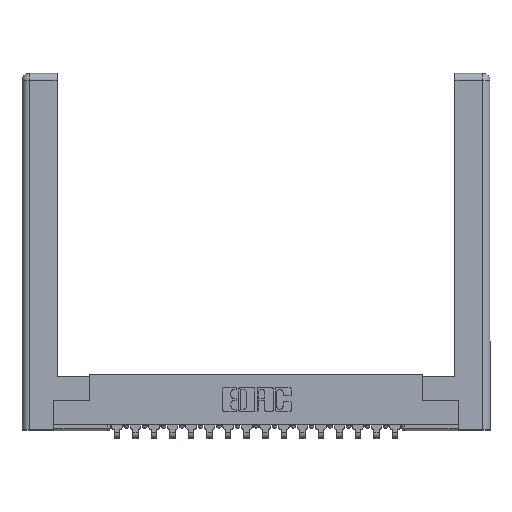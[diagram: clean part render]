
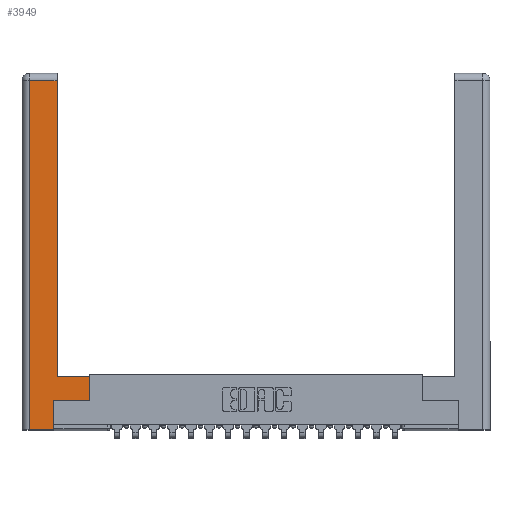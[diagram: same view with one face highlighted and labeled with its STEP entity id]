
A CAD part, top view. The second image highlights one B-rep face of the part: STEP entity #3949.
In plain terms, the highlighted planar face has unit normal (0, 0, 1).
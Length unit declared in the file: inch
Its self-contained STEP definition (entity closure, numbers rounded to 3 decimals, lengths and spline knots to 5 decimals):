
#124 = VECTOR ( 'NONE', #1855, 39.37008 ) ;
#143 = CARTESIAN_POINT ( 'NONE',  ( 0.0615, 2.94, 0. ) ) ;
#228 = VERTEX_POINT ( 'NONE', #16128 ) ;
#897 = EDGE_CURVE ( 'NONE', #4246, #228, #5765, .T. ) ;
#951 = LINE ( 'NONE', #14610, #17757 ) ;
#1146 = EDGE_CURVE ( 'NONE', #18111, #5167, #15781, .T. ) ;
#1274 = CARTESIAN_POINT ( 'NONE',  ( 0.565, 0.45, 0. ) ) ;
#1351 = VECTOR ( 'NONE', #16225, 39.37008 ) ;
#1815 = VERTEX_POINT ( 'NONE', #15613 ) ;
#1855 = DIRECTION ( 'NONE',  ( 0., 1., 0. ) ) ;
#2026 = CARTESIAN_POINT ( 'NONE',  ( 0.265, 0., 0. ) ) ;
#2850 = VECTOR ( 'NONE', #12088, 39.37008 ) ;
#3508 = CARTESIAN_POINT ( 'NONE',  ( 0., 0., 0. ) ) ;
#3619 = EDGE_CURVE ( 'NONE', #10464, #18111, #951, .T. ) ;
#3907 = ORIENTED_EDGE ( 'NONE', *, *, #15767, .T. ) ;
#3949 = ADVANCED_FACE ( 'NONE', ( #6427 ), #17150, .F. ) ;
#4221 = DIRECTION ( 'NONE',  ( 1., 0., 0. ) ) ;
#4240 = VERTEX_POINT ( 'NONE', #12368 ) ;
#4246 = VERTEX_POINT ( 'NONE', #13766 ) ;
#4341 = CARTESIAN_POINT ( 'NONE',  ( 0.265, 0.245, 0. ) ) ;
#4457 = EDGE_LOOP ( 'NONE', ( #18686, #18593, #3907, #13509, #6131, #5398, #11695, #14628 ) ) ;
#4713 = DIRECTION ( 'NONE',  ( -1., 0., 0. ) ) ;
#5167 = VERTEX_POINT ( 'NONE', #4341 ) ;
#5346 = LINE ( 'NONE', #6762, #124 ) ;
#5398 = ORIENTED_EDGE ( 'NONE', *, *, #19373, .T. ) ;
#5441 = DIRECTION ( 'NONE',  ( 0., 1., 0. ) ) ;
#5765 = LINE ( 'NONE', #1274, #13965 ) ;
#5906 = EDGE_CURVE ( 'NONE', #228, #1815, #11993, .T. ) ;
#6131 = ORIENTED_EDGE ( 'NONE', *, *, #1146, .T. ) ;
#6390 = AXIS2_PLACEMENT_3D ( 'NONE', #3508, #12706, #4713 ) ;
#6427 = FACE_OUTER_BOUND ( 'NONE', #4457, .T. ) ;
#6500 = EDGE_CURVE ( 'NONE', #15437, #4240, #12420, .T. ) ;
#6754 = CARTESIAN_POINT ( 'NONE',  ( 0.265, 0.245, 0. ) ) ;
#6762 = CARTESIAN_POINT ( 'NONE',  ( 0.295, 3., 0. ) ) ;
#7241 = DIRECTION ( 'NONE',  ( 1., 0., 0. ) ) ;
#7401 = CARTESIAN_POINT ( 'NONE',  ( 0.295, 0.45, 0. ) ) ;
#9635 = CARTESIAN_POINT ( 'NONE',  ( 0.0615, 0., 0. ) ) ;
#10326 = VECTOR ( 'NONE', #5441, 39.37008 ) ;
#10340 = CARTESIAN_POINT ( 'NONE',  ( 0.565, 0.245, 0. ) ) ;
#10464 = VERTEX_POINT ( 'NONE', #9635 ) ;
#11695 = ORIENTED_EDGE ( 'NONE', *, *, #897, .T. ) ;
#11863 = DIRECTION ( 'NONE',  ( 0., 1., 0. ) ) ;
#11993 = LINE ( 'NONE', #7401, #2850 ) ;
#12088 = DIRECTION ( 'NONE',  ( -1., 0., 0. ) ) ;
#12323 = DIRECTION ( 'NONE',  ( -1., 0., 0. ) ) ;
#12368 = CARTESIAN_POINT ( 'NONE',  ( 0.0615, 2.94, 0. ) ) ;
#12420 = LINE ( 'NONE', #143, #14371 ) ;
#12706 = DIRECTION ( 'NONE',  ( 0., 0., -1. ) ) ;
#13509 = ORIENTED_EDGE ( 'NONE', *, *, #3619, .T. ) ;
#13766 = CARTESIAN_POINT ( 'NONE',  ( 0.565, 0.245, 0. ) ) ;
#13965 = VECTOR ( 'NONE', #11863, 39.37008 ) ;
#14371 = VECTOR ( 'NONE', #12323, 39.37008 ) ;
#14610 = CARTESIAN_POINT ( 'NONE',  ( 0.265, 0., 0. ) ) ;
#14628 = ORIENTED_EDGE ( 'NONE', *, *, #5906, .T. ) ;
#14689 = LINE ( 'NONE', #10340, #15436 ) ;
#15436 = VECTOR ( 'NONE', #4221, 39.37008 ) ;
#15437 = VERTEX_POINT ( 'NONE', #15457 ) ;
#15457 = CARTESIAN_POINT ( 'NONE',  ( 0.295, 2.94, 0. ) ) ;
#15613 = CARTESIAN_POINT ( 'NONE',  ( 0.295, 0.45, 0. ) ) ;
#15767 = EDGE_CURVE ( 'NONE', #4240, #10464, #16532, .T. ) ;
#15781 = LINE ( 'NONE', #6754, #10326 ) ;
#16127 = CARTESIAN_POINT ( 'NONE',  ( 0.0615, 0., 0. ) ) ;
#16128 = CARTESIAN_POINT ( 'NONE',  ( 0.565, 0.45, 0. ) ) ;
#16225 = DIRECTION ( 'NONE',  ( 0., -1., 0. ) ) ;
#16532 = LINE ( 'NONE', #16127, #1351 ) ;
#17150 = PLANE ( 'NONE',  #6390 ) ;
#17722 = EDGE_CURVE ( 'NONE', #1815, #15437, #5346, .T. ) ;
#17757 = VECTOR ( 'NONE', #7241, 39.37008 ) ;
#18111 = VERTEX_POINT ( 'NONE', #2026 ) ;
#18593 = ORIENTED_EDGE ( 'NONE', *, *, #6500, .T. ) ;
#18686 = ORIENTED_EDGE ( 'NONE', *, *, #17722, .T. ) ;
#19373 = EDGE_CURVE ( 'NONE', #5167, #4246, #14689, .T. ) ;
